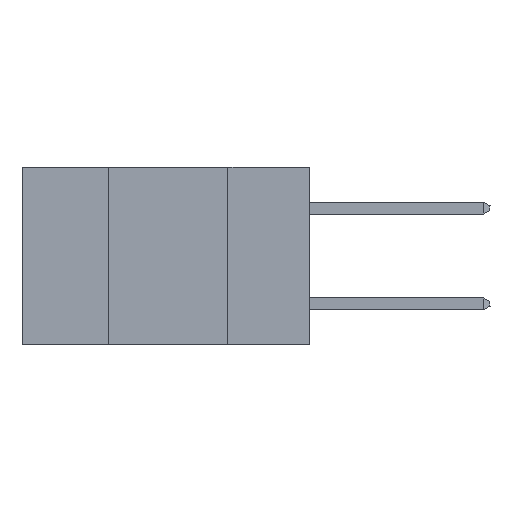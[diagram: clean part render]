
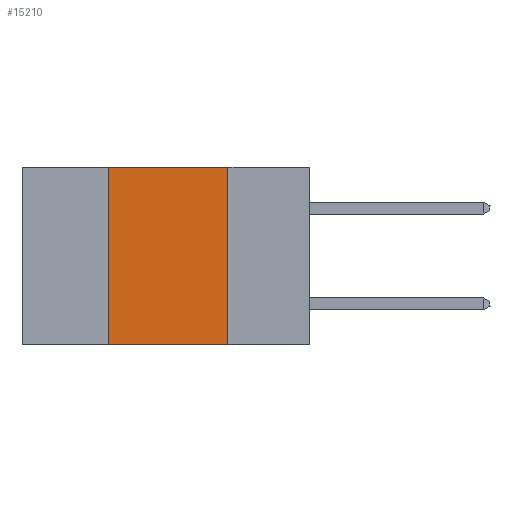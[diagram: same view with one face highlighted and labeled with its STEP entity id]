
A CAD part, left-side view. The second image highlights one B-rep face of the part: STEP entity #15210.
In plain terms, the highlighted planar face has unit normal (-1, 0, 0).
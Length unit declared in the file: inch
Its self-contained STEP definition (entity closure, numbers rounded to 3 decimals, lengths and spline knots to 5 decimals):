
#316 = VERTEX_POINT ( 'NONE', #23518 ) ;
#941 = DIRECTION ( 'NONE',  ( 0., -1., 0. ) ) ;
#1244 = VERTEX_POINT ( 'NONE', #19981 ) ;
#2083 = DIRECTION ( 'NONE',  ( 0., 0., -1. ) ) ;
#2348 = CARTESIAN_POINT ( 'NONE',  ( 0., 0.17, 0. ) ) ;
#2780 = ORIENTED_EDGE ( 'NONE', *, *, #31333, .T. ) ;
#3669 = CARTESIAN_POINT ( 'NONE',  ( 0., 0.6, 0. ) ) ;
#4288 = ORIENTED_EDGE ( 'NONE', *, *, #10389, .F. ) ;
#4756 = DIRECTION ( 'NONE',  ( 1., 0., 0. ) ) ;
#7548 = VECTOR ( 'NONE', #15332, 39.37008 ) ;
#9307 = VECTOR ( 'NONE', #14514, 39.37008 ) ;
#10389 = EDGE_CURVE ( 'NONE', #10803, #316, #36669, .T. ) ;
#10803 = VERTEX_POINT ( 'NONE', #13726 ) ;
#13226 = CARTESIAN_POINT ( 'NONE',  ( 0., 0.6, 0. ) ) ;
#13247 = LINE ( 'NONE', #2348, #14694 ) ;
#13726 = CARTESIAN_POINT ( 'NONE',  ( 0., 0.42, 0. ) ) ;
#13993 = CARTESIAN_POINT ( 'NONE',  ( 0., 0.42, -0.37 ) ) ;
#14322 = ORIENTED_EDGE ( 'NONE', *, *, #30473, .F. ) ;
#14514 = DIRECTION ( 'NONE',  ( 0., 0., 1. ) ) ;
#14694 = VECTOR ( 'NONE', #2083, 39.37008 ) ;
#15210 = ADVANCED_FACE ( 'NONE', ( #25842 ), #22687, .F. ) ;
#15332 = DIRECTION ( 'NONE',  ( 0., -1., 0. ) ) ;
#15967 = DIRECTION ( 'NONE',  ( 0., 0., -1. ) ) ;
#17324 = VECTOR ( 'NONE', #941, 39.37008 ) ;
#17353 = LINE ( 'NONE', #17414, #9307 ) ;
#17414 = CARTESIAN_POINT ( 'NONE',  ( 0., 0.42, 0. ) ) ;
#18788 = CARTESIAN_POINT ( 'NONE',  ( 0., 0.6, -0.37 ) ) ;
#19981 = CARTESIAN_POINT ( 'NONE',  ( 0., 0.17, -0.37 ) ) ;
#20693 = EDGE_LOOP ( 'NONE', ( #32118, #4288, #14322, #2780 ) ) ;
#22687 = PLANE ( 'NONE',  #35697 ) ;
#23518 = CARTESIAN_POINT ( 'NONE',  ( 0., 0.17, 0. ) ) ;
#25842 = FACE_OUTER_BOUND ( 'NONE', #20693, .T. ) ;
#28380 = EDGE_CURVE ( 'NONE', #316, #1244, #13247, .T. ) ;
#30473 = EDGE_CURVE ( 'NONE', #35039, #10803, #17353, .T. ) ;
#31333 = EDGE_CURVE ( 'NONE', #35039, #1244, #32346, .T. ) ;
#32118 = ORIENTED_EDGE ( 'NONE', *, *, #28380, .F. ) ;
#32346 = LINE ( 'NONE', #18788, #17324 ) ;
#35039 = VERTEX_POINT ( 'NONE', #13993 ) ;
#35697 = AXIS2_PLACEMENT_3D ( 'NONE', #13226, #4756, #15967 ) ;
#36669 = LINE ( 'NONE', #3669, #7548 ) ;
